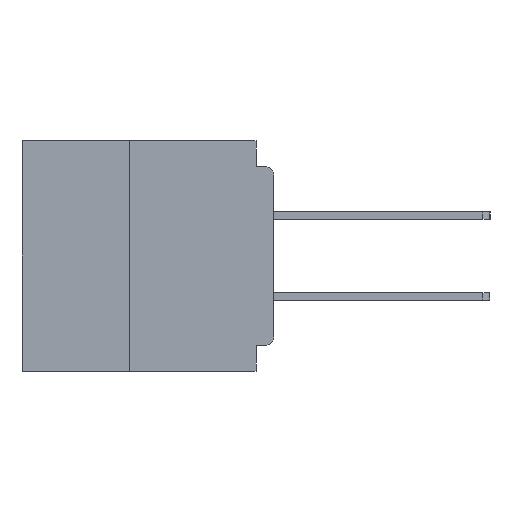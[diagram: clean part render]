
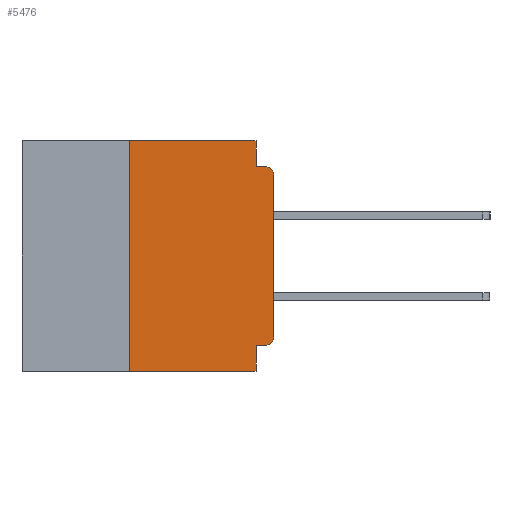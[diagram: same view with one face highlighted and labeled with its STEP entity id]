
A CAD part, left-side view. The second image highlights one B-rep face of the part: STEP entity #5476.
In plain terms, the highlighted planar face has unit normal (-1, 0, 0).
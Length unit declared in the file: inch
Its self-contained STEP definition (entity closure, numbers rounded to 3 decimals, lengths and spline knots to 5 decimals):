
#6 = DIRECTION ( 'NONE',  ( 0., -1., 0. ) ) ;
#478 = DIRECTION ( 'NONE',  ( 0., 0., -1. ) ) ;
#3564 = AXIS2_PLACEMENT_3D ( 'NONE', #35351, #10269, #39531 ) ;
#3653 = CIRCLE ( 'NONE', #3564, 0.015 ) ;
#4336 = LINE ( 'NONE', #7166, #36430 ) ;
#4486 = EDGE_CURVE ( 'NONE', #21118, #40986, #3653, .T. ) ;
#4784 = DIRECTION ( 'NONE',  ( -1., 0., 0. ) ) ;
#4922 = CARTESIAN_POINT ( 'NONE',  ( 0., 0., -0.34 ) ) ;
#4955 = ORIENTED_EDGE ( 'NONE', *, *, #16223, .F. ) ;
#5317 = CARTESIAN_POINT ( 'NONE',  ( 0., 0.031, 0. ) ) ;
#5476 = ADVANCED_FACE ( 'NONE', ( #42799 ), #9452, .F. ) ;
#5531 = CARTESIAN_POINT ( 'NONE',  ( 0., 0.015, -0.355 ) ) ;
#6991 = VECTOR ( 'NONE', #47689, 39.37008 ) ;
#7166 = CARTESIAN_POINT ( 'NONE',  ( 0., 0.437, -0.4 ) ) ;
#9452 = PLANE ( 'NONE',  #53611 ) ;
#9744 = EDGE_LOOP ( 'NONE', ( #30293, #48375, #12907, #36472, #49192, #40868, #19312, #4955, #10552, #32186 ) ) ;
#10269 = DIRECTION ( 'NONE',  ( -1., 0., 0. ) ) ;
#10552 = ORIENTED_EDGE ( 'NONE', *, *, #24216, .F. ) ;
#12907 = ORIENTED_EDGE ( 'NONE', *, *, #13238, .F. ) ;
#13238 = EDGE_CURVE ( 'NONE', #30242, #40986, #47223, .T. ) ;
#13637 = DIRECTION ( 'NONE',  ( 0., 0., -1. ) ) ;
#13652 = DIRECTION ( 'NONE',  ( 1., 0., 0. ) ) ;
#13868 = EDGE_CURVE ( 'NONE', #27383, #18142, #44466, .T. ) ;
#13916 = VECTOR ( 'NONE', #6, 39.37008 ) ;
#13939 = VERTEX_POINT ( 'NONE', #5317 ) ;
#14067 = CARTESIAN_POINT ( 'NONE',  ( 0., 0.25, -0.4 ) ) ;
#14290 = CARTESIAN_POINT ( 'NONE',  ( 0., 0.437, 0. ) ) ;
#14332 = CARTESIAN_POINT ( 'NONE',  ( 0., 0., 0. ) ) ;
#14448 = LINE ( 'NONE', #17414, #21623 ) ;
#15855 = EDGE_CURVE ( 'NONE', #18142, #21118, #37749, .T. ) ;
#16223 = EDGE_CURVE ( 'NONE', #53121, #29474, #17516, .T. ) ;
#16404 = EDGE_CURVE ( 'NONE', #53083, #13939, #19427, .T. ) ;
#17414 = CARTESIAN_POINT ( 'NONE',  ( 0., 0., -0.355 ) ) ;
#17516 = LINE ( 'NONE', #38265, #48184 ) ;
#18142 = VERTEX_POINT ( 'NONE', #4922 ) ;
#18416 = AXIS2_PLACEMENT_3D ( 'NONE', #29873, #4784, #34103 ) ;
#19312 = ORIENTED_EDGE ( 'NONE', *, *, #29439, .T. ) ;
#19427 = LINE ( 'NONE', #14290, #6991 ) ;
#19965 = CARTESIAN_POINT ( 'NONE',  ( 0., 0.031, -0.4 ) ) ;
#20262 = LINE ( 'NONE', #43233, #30095 ) ;
#21118 = VERTEX_POINT ( 'NONE', #35464 ) ;
#21603 = DIRECTION ( 'NONE',  ( 0., 1., 0. ) ) ;
#21623 = VECTOR ( 'NONE', #21603, 39.37008 ) ;
#24216 = EDGE_CURVE ( 'NONE', #27383, #53121, #14448, .T. ) ;
#24751 = EDGE_CURVE ( 'NONE', #26050, #53083, #20262, .T. ) ;
#26050 = VERTEX_POINT ( 'NONE', #14067 ) ;
#27383 = VERTEX_POINT ( 'NONE', #5531 ) ;
#27997 = CARTESIAN_POINT ( 'NONE',  ( 0., 0.031, -0.355 ) ) ;
#29439 = EDGE_CURVE ( 'NONE', #26050, #29474, #4336, .T. ) ;
#29474 = VERTEX_POINT ( 'NONE', #19965 ) ;
#29873 = CARTESIAN_POINT ( 'NONE',  ( 0., 0.015, -0.34 ) ) ;
#30095 = VECTOR ( 'NONE', #39056, 39.37008 ) ;
#30242 = VERTEX_POINT ( 'NONE', #37494 ) ;
#30293 = ORIENTED_EDGE ( 'NONE', *, *, #15855, .T. ) ;
#30301 = CARTESIAN_POINT ( 'NONE',  ( 0., 0.437, 0. ) ) ;
#32186 = ORIENTED_EDGE ( 'NONE', *, *, #13868, .T. ) ;
#33837 = VECTOR ( 'NONE', #51867, 39.37008 ) ;
#34103 = DIRECTION ( 'NONE',  ( 0., 0., -1. ) ) ;
#35351 = CARTESIAN_POINT ( 'NONE',  ( 0., 0.015, -0.06 ) ) ;
#35464 = CARTESIAN_POINT ( 'NONE',  ( 0., 0., -0.06 ) ) ;
#36130 = LINE ( 'NONE', #42858, #48488 ) ;
#36430 = VECTOR ( 'NONE', #40648, 39.37008 ) ;
#36472 = ORIENTED_EDGE ( 'NONE', *, *, #40060, .F. ) ;
#37494 = CARTESIAN_POINT ( 'NONE',  ( 0., 0.031, -0.045 ) ) ;
#37749 = LINE ( 'NONE', #14332, #33837 ) ;
#38265 = CARTESIAN_POINT ( 'NONE',  ( 0., 0.031, -0.4 ) ) ;
#39056 = DIRECTION ( 'NONE',  ( 0., 0., 1. ) ) ;
#39531 = DIRECTION ( 'NONE',  ( 0., 0., -1. ) ) ;
#40060 = EDGE_CURVE ( 'NONE', #13939, #30242, #36130, .T. ) ;
#40403 = CARTESIAN_POINT ( 'NONE',  ( 0., 0.25, 0. ) ) ;
#40648 = DIRECTION ( 'NONE',  ( 0., -1., 0. ) ) ;
#40868 = ORIENTED_EDGE ( 'NONE', *, *, #24751, .F. ) ;
#40986 = VERTEX_POINT ( 'NONE', #41349 ) ;
#41349 = CARTESIAN_POINT ( 'NONE',  ( 0., 0.015, -0.045 ) ) ;
#42799 = FACE_OUTER_BOUND ( 'NONE', #9744, .T. ) ;
#42858 = CARTESIAN_POINT ( 'NONE',  ( 0., 0.031, 0. ) ) ;
#42871 = DIRECTION ( 'NONE',  ( 0., 0., -1. ) ) ;
#43233 = CARTESIAN_POINT ( 'NONE',  ( 0., 0.25, -0.4 ) ) ;
#44466 = CIRCLE ( 'NONE', #18416, 0.015 ) ;
#47223 = LINE ( 'NONE', #50115, #13916 ) ;
#47689 = DIRECTION ( 'NONE',  ( 0., -1., 0. ) ) ;
#48184 = VECTOR ( 'NONE', #478, 39.37008 ) ;
#48375 = ORIENTED_EDGE ( 'NONE', *, *, #4486, .T. ) ;
#48488 = VECTOR ( 'NONE', #13637, 39.37008 ) ;
#49192 = ORIENTED_EDGE ( 'NONE', *, *, #16404, .F. ) ;
#50115 = CARTESIAN_POINT ( 'NONE',  ( 0., 0., -0.045 ) ) ;
#51867 = DIRECTION ( 'NONE',  ( 0., 0., 1. ) ) ;
#53083 = VERTEX_POINT ( 'NONE', #40403 ) ;
#53121 = VERTEX_POINT ( 'NONE', #27997 ) ;
#53611 = AXIS2_PLACEMENT_3D ( 'NONE', #30301, #13652, #42871 ) ;
